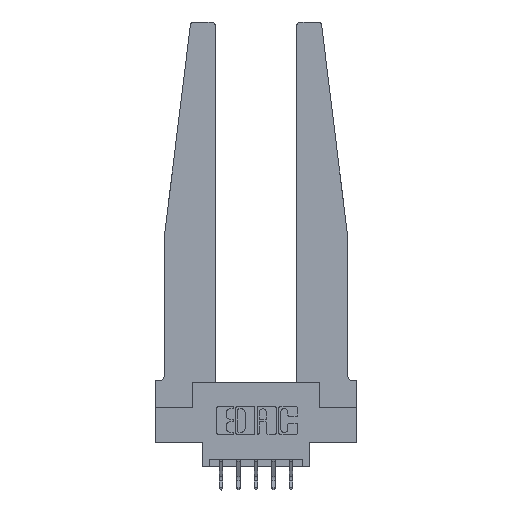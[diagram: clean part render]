
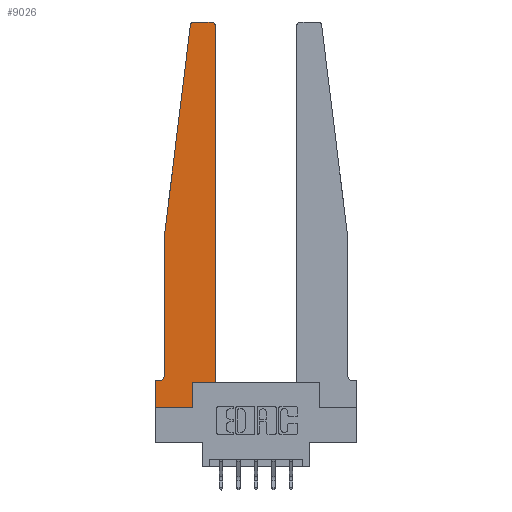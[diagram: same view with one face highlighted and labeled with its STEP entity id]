
A CAD part, top view. The second image highlights one B-rep face of the part: STEP entity #9026.
In plain terms, the highlighted planar face has unit normal (0, 0, 1).
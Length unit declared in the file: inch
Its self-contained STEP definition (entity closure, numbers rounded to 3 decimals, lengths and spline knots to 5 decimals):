
#106 = CARTESIAN_POINT ( 'NONE',  ( 0.015, 0.2375, 0.37 ) ) ;
#137 = DIRECTION ( 'NONE',  ( 0., 0., 1. ) ) ;
#299 = CARTESIAN_POINT ( 'NONE',  ( 0.065, 1.25, 0.37 ) ) ;
#324 = ORIENTED_EDGE ( 'NONE', *, *, #5409, .T. ) ;
#362 = DIRECTION ( 'NONE',  ( 0., 0., 1. ) ) ;
#417 = CARTESIAN_POINT ( 'NONE',  ( 0.2605, 0., 0.37 ) ) ;
#482 = VERTEX_POINT ( 'NONE', #5024 ) ;
#552 = EDGE_CURVE ( 'NONE', #9959, #6405, #2943, .T. ) ;
#591 = DIRECTION ( 'NONE',  ( 0., 1., 0. ) ) ;
#625 = VECTOR ( 'NONE', #2012, 39.37008 ) ;
#660 = EDGE_CURVE ( 'NONE', #11349, #482, #12032, .T. ) ;
#688 = ORIENTED_EDGE ( 'NONE', *, *, #12593, .T. ) ;
#757 = VECTOR ( 'NONE', #835, 39.37008 ) ;
#816 = VERTEX_POINT ( 'NONE', #8267 ) ;
#835 = DIRECTION ( 'NONE',  ( 0., -1., 0. ) ) ;
#939 = LINE ( 'NONE', #3995, #9671 ) ;
#1255 = ORIENTED_EDGE ( 'NONE', *, *, #5750, .T. ) ;
#1475 = LINE ( 'NONE', #4618, #5767 ) ;
#1628 = VERTEX_POINT ( 'NONE', #11222 ) ;
#2012 = DIRECTION ( 'NONE',  ( 1., 0., 0. ) ) ;
#2063 = VECTOR ( 'NONE', #591, 39.37008 ) ;
#2253 = DIRECTION ( 'NONE',  ( -0.122, -0.992, 0. ) ) ;
#2472 = VERTEX_POINT ( 'NONE', #7492 ) ;
#2514 = CIRCLE ( 'NONE', #2971, 0.03 ) ;
#2544 = LINE ( 'NONE', #13097, #10326 ) ;
#2677 = DIRECTION ( 'NONE',  ( 1., 0., 0. ) ) ;
#2700 = VERTEX_POINT ( 'NONE', #13078 ) ;
#2770 = DIRECTION ( 'NONE',  ( -1., 0., 0. ) ) ;
#2813 = LINE ( 'NONE', #4899, #2063 ) ;
#2943 = LINE ( 'NONE', #10431, #625 ) ;
#2971 = AXIS2_PLACEMENT_3D ( 'NONE', #7468, #137, #12910 ) ;
#2972 = VERTEX_POINT ( 'NONE', #10639 ) ;
#2975 = LINE ( 'NONE', #4839, #10127 ) ;
#3230 = DIRECTION ( 'NONE',  ( -1., 0., 0. ) ) ;
#3786 = ORIENTED_EDGE ( 'NONE', *, *, #11354, .T. ) ;
#3995 = CARTESIAN_POINT ( 'NONE',  ( 0.425, 0.18, 0.37 ) ) ;
#4527 = DIRECTION ( 'NONE',  ( 1., 0., 0. ) ) ;
#4552 = ORIENTED_EDGE ( 'NONE', *, *, #11804, .T. ) ;
#4594 = EDGE_CURVE ( 'NONE', #1628, #8212, #2544, .T. ) ;
#4618 = CARTESIAN_POINT ( 'NONE',  ( 0.065, 1.25, 0.37 ) ) ;
#4693 = ORIENTED_EDGE ( 'NONE', *, *, #12067, .T. ) ;
#4839 = CARTESIAN_POINT ( 'NONE',  ( 0.25, 2.75, 0.37 ) ) ;
#4899 = CARTESIAN_POINT ( 'NONE',  ( 0.2605, 0.18, 0.37 ) ) ;
#5024 = CARTESIAN_POINT ( 'NONE',  ( 0.065, 0.2375, 0.37 ) ) ;
#5409 = EDGE_CURVE ( 'NONE', #2700, #9441, #6337, .T. ) ;
#5750 = EDGE_CURVE ( 'NONE', #6177, #1628, #9699, .T. ) ;
#5767 = VECTOR ( 'NONE', #2253, 39.37008 ) ;
#5951 = ORIENTED_EDGE ( 'NONE', *, *, #552, .T. ) ;
#6177 = VERTEX_POINT ( 'NONE', #6666 ) ;
#6337 = CIRCLE ( 'NONE', #13027, 0.03 ) ;
#6405 = VERTEX_POINT ( 'NONE', #10427 ) ;
#6579 = EDGE_LOOP ( 'NONE', ( #4693, #4552, #11423, #8968, #688, #7862, #1255, #9680, #7954, #5951, #3786, #324 ) ) ;
#6666 = CARTESIAN_POINT ( 'NONE',  ( 0., 0.1875, 0.37 ) ) ;
#6748 = PLANE ( 'NONE',  #12909 ) ;
#6980 = EDGE_CURVE ( 'NONE', #816, #6177, #10189, .T. ) ;
#7011 = DIRECTION ( 'NONE',  ( 1., 0., 0. ) ) ;
#7468 = CARTESIAN_POINT ( 'NONE',  ( 0.27653, 2.72, 0.37 ) ) ;
#7492 = CARTESIAN_POINT ( 'NONE',  ( 0.24675, 2.72367, 0.37 ) ) ;
#7862 = ORIENTED_EDGE ( 'NONE', *, *, #6980, .T. ) ;
#7892 = CARTESIAN_POINT ( 'NONE',  ( 0.395, 2.75, 0.37 ) ) ;
#7954 = ORIENTED_EDGE ( 'NONE', *, *, #12498, .T. ) ;
#8140 = AXIS2_PLACEMENT_3D ( 'NONE', #106, #11558, #3230 ) ;
#8212 = VERTEX_POINT ( 'NONE', #417 ) ;
#8267 = CARTESIAN_POINT ( 'NONE',  ( 0.015, 0.1875, 0.37 ) ) ;
#8355 = VECTOR ( 'NONE', #2770, 39.37008 ) ;
#8849 = FACE_OUTER_BOUND ( 'NONE', #6579, .T. ) ;
#8968 = ORIENTED_EDGE ( 'NONE', *, *, #660, .T. ) ;
#9005 = CARTESIAN_POINT ( 'NONE',  ( 0.065, 0.1875, 0.37 ) ) ;
#9026 = ADVANCED_FACE ( 'NONE', ( #8849 ), #6748, .T. ) ;
#9441 = VERTEX_POINT ( 'NONE', #7892 ) ;
#9671 = VECTOR ( 'NONE', #12671, 39.37008 ) ;
#9680 = ORIENTED_EDGE ( 'NONE', *, *, #4594, .T. ) ;
#9699 = LINE ( 'NONE', #12765, #757 ) ;
#9959 = VERTEX_POINT ( 'NONE', #10392 ) ;
#10127 = VECTOR ( 'NONE', #13327, 39.37008 ) ;
#10189 = LINE ( 'NONE', #9005, #8355 ) ;
#10215 = EDGE_CURVE ( 'NONE', #2472, #11349, #1475, .T. ) ;
#10326 = VECTOR ( 'NONE', #2677, 39.37008 ) ;
#10392 = CARTESIAN_POINT ( 'NONE',  ( 0.2605, 0.18, 0.37 ) ) ;
#10427 = CARTESIAN_POINT ( 'NONE',  ( 0.425, 0.18, 0.37 ) ) ;
#10431 = CARTESIAN_POINT ( 'NONE',  ( 0.425, 0.18, 0.37 ) ) ;
#10451 = VECTOR ( 'NONE', #12104, 39.37008 ) ;
#10504 = CARTESIAN_POINT ( 'NONE',  ( 0.065, 1.25, 0.37 ) ) ;
#10639 = CARTESIAN_POINT ( 'NONE',  ( 0.27653, 2.75, 0.37 ) ) ;
#10997 = CARTESIAN_POINT ( 'NONE',  ( 0., 0.1875, 0.37 ) ) ;
#11222 = CARTESIAN_POINT ( 'NONE',  ( 0., 0., 0.37 ) ) ;
#11349 = VERTEX_POINT ( 'NONE', #10504 ) ;
#11354 = EDGE_CURVE ( 'NONE', #6405, #2700, #939, .T. ) ;
#11423 = ORIENTED_EDGE ( 'NONE', *, *, #10215, .T. ) ;
#11471 = CIRCLE ( 'NONE', #8140, 0.05 ) ;
#11558 = DIRECTION ( 'NONE',  ( 0., 0., -1. ) ) ;
#11804 = EDGE_CURVE ( 'NONE', #2972, #2472, #2514, .T. ) ;
#12032 = LINE ( 'NONE', #299, #10451 ) ;
#12067 = EDGE_CURVE ( 'NONE', #9441, #2972, #2975, .T. ) ;
#12096 = CARTESIAN_POINT ( 'NONE',  ( 0.395, 2.72, 0.37 ) ) ;
#12104 = DIRECTION ( 'NONE',  ( 0., -1., 0. ) ) ;
#12498 = EDGE_CURVE ( 'NONE', #8212, #9959, #2813, .T. ) ;
#12593 = EDGE_CURVE ( 'NONE', #482, #816, #11471, .T. ) ;
#12671 = DIRECTION ( 'NONE',  ( 0., 1., 0. ) ) ;
#12765 = CARTESIAN_POINT ( 'NONE',  ( 0., 0., 0.37 ) ) ;
#12909 = AXIS2_PLACEMENT_3D ( 'NONE', #10997, #13090, #7011 ) ;
#12910 = DIRECTION ( 'NONE',  ( 1., 0., 0. ) ) ;
#13027 = AXIS2_PLACEMENT_3D ( 'NONE', #12096, #362, #4527 ) ;
#13078 = CARTESIAN_POINT ( 'NONE',  ( 0.425, 2.72, 0.37 ) ) ;
#13090 = DIRECTION ( 'NONE',  ( 0., 0., 1. ) ) ;
#13097 = CARTESIAN_POINT ( 'NONE',  ( 0., 0., 0.37 ) ) ;
#13327 = DIRECTION ( 'NONE',  ( -1., 0., 0. ) ) ;
